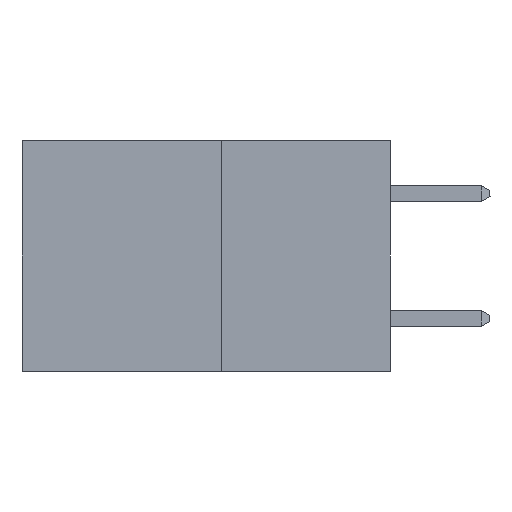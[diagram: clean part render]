
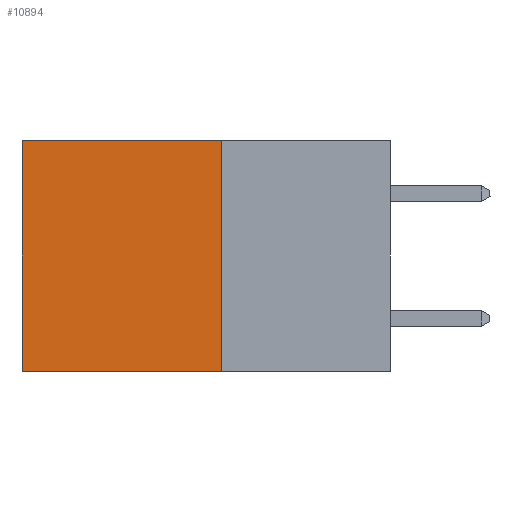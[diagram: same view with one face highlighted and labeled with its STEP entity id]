
A CAD part, left-side view. The second image highlights one B-rep face of the part: STEP entity #10894.
In plain terms, the highlighted planar face has unit normal (-1, 0, 0).
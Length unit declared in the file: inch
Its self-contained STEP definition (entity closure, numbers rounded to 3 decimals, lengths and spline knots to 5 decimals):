
#356 = VERTEX_POINT ( 'NONE', #3455 ) ;
#700 = DIRECTION ( 'NONE',  ( 0., 0., -1. ) ) ;
#1197 = EDGE_CURVE ( 'NONE', #13029, #14900, #15626, .T. ) ;
#1960 = DIRECTION ( 'NONE',  ( 0., 1., 0. ) ) ;
#2665 = CARTESIAN_POINT ( 'NONE',  ( 0.277, 0.27, -0.37 ) ) ;
#2680 = EDGE_CURVE ( 'NONE', #13029, #13441, #4653, .T. ) ;
#2826 = VECTOR ( 'NONE', #12652, 39.37008 ) ;
#3455 = CARTESIAN_POINT ( 'NONE',  ( 0.277, 0.59, -0.37 ) ) ;
#3583 = DIRECTION ( 'NONE',  ( 1., 0., 0. ) ) ;
#3686 = CARTESIAN_POINT ( 'NONE',  ( 0.277, 0.59, 0. ) ) ;
#4653 = LINE ( 'NONE', #5956, #14246 ) ;
#4909 = CARTESIAN_POINT ( 'NONE',  ( 0.277, 0.27, -0.37 ) ) ;
#5956 = CARTESIAN_POINT ( 'NONE',  ( 0.277, 0.27, 0. ) ) ;
#6383 = CARTESIAN_POINT ( 'NONE',  ( 0.277, 0.59, -0.37 ) ) ;
#7335 = CARTESIAN_POINT ( 'NONE',  ( 0.277, 0.27, -0.37 ) ) ;
#7651 = LINE ( 'NONE', #6383, #13499 ) ;
#8498 = ORIENTED_EDGE ( 'NONE', *, *, #1197, .F. ) ;
#9251 = CARTESIAN_POINT ( 'NONE',  ( 0.277, 0.27, 0. ) ) ;
#9455 = LINE ( 'NONE', #2665, #2826 ) ;
#10344 = EDGE_CURVE ( 'NONE', #14900, #356, #9455, .T. ) ;
#10428 = EDGE_LOOP ( 'NONE', ( #15959, #15577, #8498, #15421 ) ) ;
#10894 = ADVANCED_FACE ( 'NONE', ( #14572 ), #16038, .F. ) ;
#11031 = AXIS2_PLACEMENT_3D ( 'NONE', #7335, #3583, #12307 ) ;
#11351 = DIRECTION ( 'NONE',  ( 0., 0., -1. ) ) ;
#11878 = VECTOR ( 'NONE', #700, 39.37008 ) ;
#12307 = DIRECTION ( 'NONE',  ( 0., 0., -1. ) ) ;
#12652 = DIRECTION ( 'NONE',  ( 0., 1., 0. ) ) ;
#12959 = EDGE_CURVE ( 'NONE', #13441, #356, #7651, .T. ) ;
#13029 = VERTEX_POINT ( 'NONE', #9251 ) ;
#13441 = VERTEX_POINT ( 'NONE', #3686 ) ;
#13499 = VECTOR ( 'NONE', #11351, 39.37008 ) ;
#13875 = CARTESIAN_POINT ( 'NONE',  ( 0.277, 0.27, -0.37 ) ) ;
#14246 = VECTOR ( 'NONE', #1960, 39.37008 ) ;
#14572 = FACE_OUTER_BOUND ( 'NONE', #10428, .T. ) ;
#14900 = VERTEX_POINT ( 'NONE', #13875 ) ;
#15421 = ORIENTED_EDGE ( 'NONE', *, *, #2680, .T. ) ;
#15577 = ORIENTED_EDGE ( 'NONE', *, *, #10344, .F. ) ;
#15626 = LINE ( 'NONE', #4909, #11878 ) ;
#15959 = ORIENTED_EDGE ( 'NONE', *, *, #12959, .T. ) ;
#16038 = PLANE ( 'NONE',  #11031 ) ;
